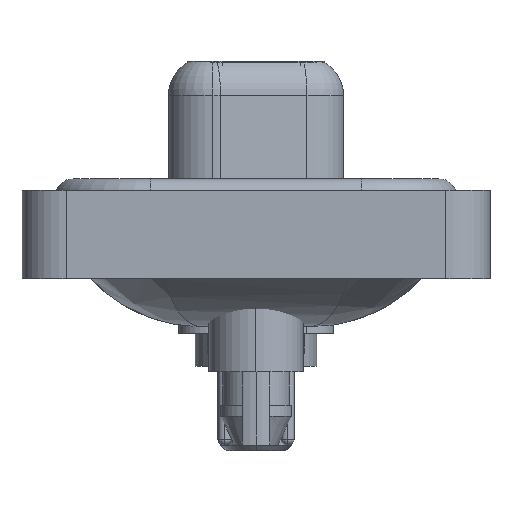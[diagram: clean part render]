
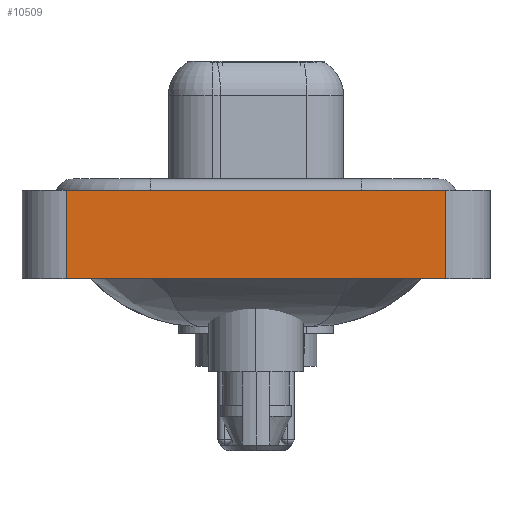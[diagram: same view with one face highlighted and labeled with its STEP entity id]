
A CAD part, left-side view. The second image highlights one B-rep face of the part: STEP entity #10509.
In plain terms, the highlighted planar face has unit normal (-1, 0, 0).
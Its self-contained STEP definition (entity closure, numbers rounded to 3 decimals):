
#810 = LINE ( 'NONE', #10797, #8863 ) ;
#2544 = ORIENTED_EDGE ( 'NONE', *, *, #13931, .F. ) ;
#2648 = ORIENTED_EDGE ( 'NONE', *, *, #19440, .T. ) ;
#2852 = DIRECTION ( 'NONE',  ( 0., 0., 1. ) ) ;
#4620 = ORIENTED_EDGE ( 'NONE', *, *, #14287, .T. ) ;
#4806 = ORIENTED_EDGE ( 'NONE', *, *, #10202, .F. ) ;
#5470 = CARTESIAN_POINT ( 'NONE',  ( -7.25, 8.55, -3.6 ) ) ;
#5646 = CARTESIAN_POINT ( 'NONE',  ( -7.25, 8.55, 0.4 ) ) ;
#6410 = VERTEX_POINT ( 'NONE', #13347 ) ;
#7623 = CARTESIAN_POINT ( 'NONE',  ( -7.25, -8.55, -3.6 ) ) ;
#7763 = DIRECTION ( 'NONE',  ( 0., 0., 1. ) ) ;
#8703 = VERTEX_POINT ( 'NONE', #20574 ) ;
#8863 = VECTOR ( 'NONE', #7763, 1000. ) ;
#9260 = VECTOR ( 'NONE', #16065, 1000. ) ;
#9481 = LINE ( 'NONE', #12520, #9260 ) ;
#9533 = CARTESIAN_POINT ( 'NONE',  ( -7.25, -8.55, 0.4 ) ) ;
#10202 = EDGE_CURVE ( 'NONE', #13749, #15896, #20698, .T. ) ;
#10509 = ADVANCED_FACE ( 'NONE', ( #19047 ), #12677, .T. ) ;
#10797 = CARTESIAN_POINT ( 'NONE',  ( -7.25, -8.55, -3.6 ) ) ;
#12357 = DIRECTION ( 'NONE',  ( 0., 0., 1. ) ) ;
#12520 = CARTESIAN_POINT ( 'NONE',  ( -7.25, -8.55, -3.6 ) ) ;
#12677 = PLANE ( 'NONE',  #17608 ) ;
#12759 = EDGE_LOOP ( 'NONE', ( #4620, #2544, #4806, #2648 ) ) ;
#13347 = CARTESIAN_POINT ( 'NONE',  ( -7.25, -8.55, -3.6 ) ) ;
#13749 = VERTEX_POINT ( 'NONE', #5470 ) ;
#13931 = EDGE_CURVE ( 'NONE', #15896, #8703, #21200, .T. ) ;
#14287 = EDGE_CURVE ( 'NONE', #6410, #8703, #810, .T. ) ;
#15896 = VERTEX_POINT ( 'NONE', #5646 ) ;
#16065 = DIRECTION ( 'NONE',  ( 0., -1., 0. ) ) ;
#17419 = DIRECTION ( 'NONE',  ( -1., 0., 0. ) ) ;
#17552 = CARTESIAN_POINT ( 'NONE',  ( -7.25, 8.55, -3.6 ) ) ;
#17595 = VECTOR ( 'NONE', #2852, 1000. ) ;
#17608 = AXIS2_PLACEMENT_3D ( 'NONE', #7623, #17419, #12357 ) ;
#19047 = FACE_OUTER_BOUND ( 'NONE', #12759, .T. ) ;
#19440 = EDGE_CURVE ( 'NONE', #13749, #6410, #9481, .T. ) ;
#20565 = VECTOR ( 'NONE', #20859, 1000. ) ;
#20574 = CARTESIAN_POINT ( 'NONE',  ( -7.25, -8.55, 0.4 ) ) ;
#20698 = LINE ( 'NONE', #17552, #17595 ) ;
#20859 = DIRECTION ( 'NONE',  ( 0., -1., 0. ) ) ;
#21200 = LINE ( 'NONE', #9533, #20565 ) ;
